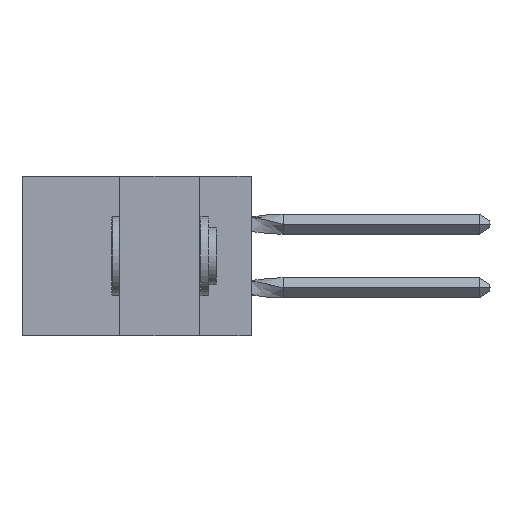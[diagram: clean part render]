
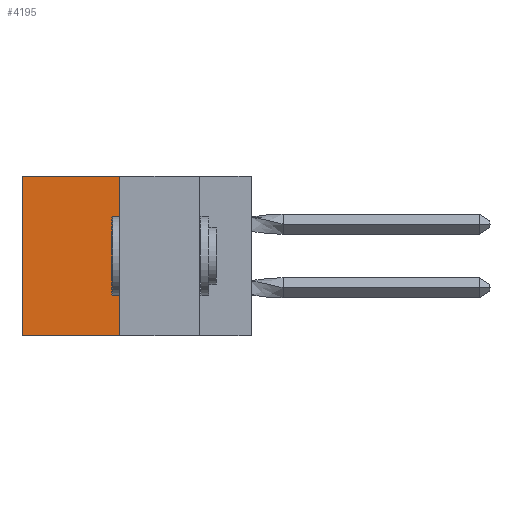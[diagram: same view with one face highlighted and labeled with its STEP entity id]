
A CAD part, left-side view. The second image highlights one B-rep face of the part: STEP entity #4195.
In plain terms, the highlighted planar face has unit normal (-1, 0, 0).
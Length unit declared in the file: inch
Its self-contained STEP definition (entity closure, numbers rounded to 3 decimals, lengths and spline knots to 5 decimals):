
#231 = DIRECTION ( 'NONE',  ( 0., 0., -1. ) ) ;
#1449 = CARTESIAN_POINT ( 'NONE',  ( 0.305, 0.72, -0.5 ) ) ;
#2368 = CARTESIAN_POINT ( 'NONE',  ( 0.305, 0.413, -0.5 ) ) ;
#3842 = VERTEX_POINT ( 'NONE', #20664 ) ;
#4195 = ADVANCED_FACE ( 'NONE', ( #6885 ), #5674, .F. ) ;
#4278 = DIRECTION ( 'NONE',  ( 0., 1., 0. ) ) ;
#4334 = VECTOR ( 'NONE', #231, 39.37008 ) ;
#5284 = VECTOR ( 'NONE', #17791, 39.37008 ) ;
#5478 = EDGE_CURVE ( 'NONE', #14815, #13808, #16782, .T. ) ;
#5674 = PLANE ( 'NONE',  #7407 ) ;
#6644 = EDGE_LOOP ( 'NONE', ( #9335, #17654, #6697, #11462 ) ) ;
#6697 = ORIENTED_EDGE ( 'NONE', *, *, #12361, .F. ) ;
#6885 = FACE_OUTER_BOUND ( 'NONE', #6644, .T. ) ;
#7407 = AXIS2_PLACEMENT_3D ( 'NONE', #15321, #17169, #18744 ) ;
#7896 = LINE ( 'NONE', #2368, #4334 ) ;
#8200 = EDGE_CURVE ( 'NONE', #13860, #14815, #16527, .T. ) ;
#9335 = ORIENTED_EDGE ( 'NONE', *, *, #5478, .T. ) ;
#11462 = ORIENTED_EDGE ( 'NONE', *, *, #8200, .T. ) ;
#12361 = EDGE_CURVE ( 'NONE', #13860, #3842, #7896, .T. ) ;
#12491 = VECTOR ( 'NONE', #4278, 39.37008 ) ;
#13674 = CARTESIAN_POINT ( 'NONE',  ( 0.305, 0.72, -0.5 ) ) ;
#13743 = CARTESIAN_POINT ( 'NONE',  ( 0.305, 0.413, 0. ) ) ;
#13808 = VERTEX_POINT ( 'NONE', #13674 ) ;
#13860 = VERTEX_POINT ( 'NONE', #13743 ) ;
#14748 = VECTOR ( 'NONE', #20376, 39.37008 ) ;
#14815 = VERTEX_POINT ( 'NONE', #14925 ) ;
#14925 = CARTESIAN_POINT ( 'NONE',  ( 0.305, 0.72, 0. ) ) ;
#15321 = CARTESIAN_POINT ( 'NONE',  ( 0.305, 0.413, -0.5 ) ) ;
#16527 = LINE ( 'NONE', #20449, #14748 ) ;
#16782 = LINE ( 'NONE', #1449, #5284 ) ;
#17169 = DIRECTION ( 'NONE',  ( 1., 0., 0. ) ) ;
#17654 = ORIENTED_EDGE ( 'NONE', *, *, #20187, .F. ) ;
#17791 = DIRECTION ( 'NONE',  ( 0., 0., -1. ) ) ;
#18620 = LINE ( 'NONE', #20885, #12491 ) ;
#18744 = DIRECTION ( 'NONE',  ( 0., 0., -1. ) ) ;
#20187 = EDGE_CURVE ( 'NONE', #3842, #13808, #18620, .T. ) ;
#20376 = DIRECTION ( 'NONE',  ( 0., 1., 0. ) ) ;
#20449 = CARTESIAN_POINT ( 'NONE',  ( 0.305, 0.413, 0. ) ) ;
#20664 = CARTESIAN_POINT ( 'NONE',  ( 0.305, 0.413, -0.5 ) ) ;
#20885 = CARTESIAN_POINT ( 'NONE',  ( 0.305, 0.413, -0.5 ) ) ;
